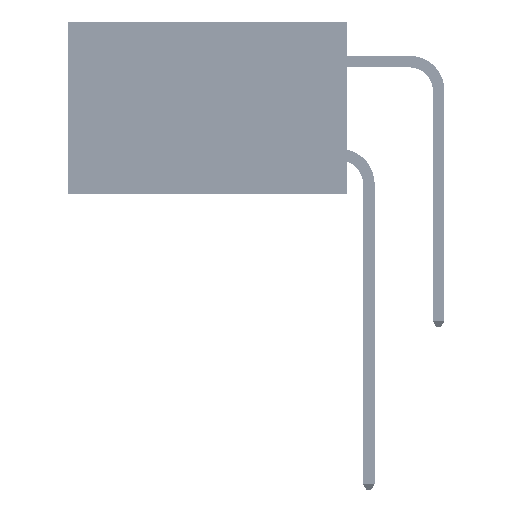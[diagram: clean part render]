
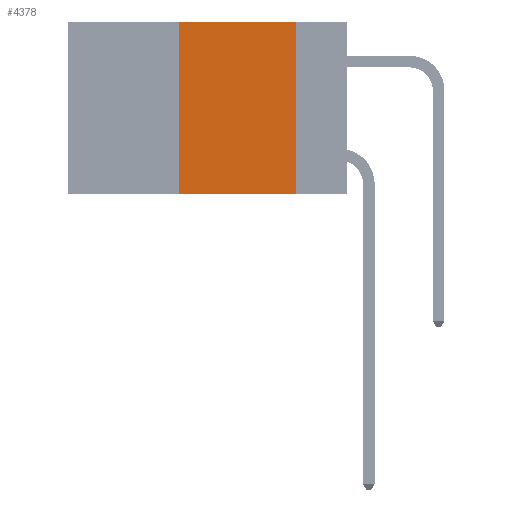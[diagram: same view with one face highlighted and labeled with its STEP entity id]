
A CAD part, left-side view. The second image highlights one B-rep face of the part: STEP entity #4378.
In plain terms, the highlighted planar face has unit normal (-1, 0, 0).
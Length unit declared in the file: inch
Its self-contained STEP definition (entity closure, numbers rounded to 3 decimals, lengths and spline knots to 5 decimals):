
#446 = AXIS2_PLACEMENT_3D ( 'NONE', #36371, #47798, #25046 ) ;
#1103 = CARTESIAN_POINT ( 'NONE',  ( 0., 0.11, 0. ) ) ;
#2057 = VERTEX_POINT ( 'NONE', #31451 ) ;
#3008 = ORIENTED_EDGE ( 'NONE', *, *, #12798, .T. ) ;
#3138 = EDGE_LOOP ( 'NONE', ( #3598, #27685, #30068, #3008 ) ) ;
#3598 = ORIENTED_EDGE ( 'NONE', *, *, #38986, .F. ) ;
#3683 = LINE ( 'NONE', #12601, #34325 ) ;
#4378 = ADVANCED_FACE ( 'NONE', ( #35462 ), #24865, .F. ) ;
#5439 = CARTESIAN_POINT ( 'NONE',  ( 0., 0.11, 0. ) ) ;
#5628 = EDGE_CURVE ( 'NONE', #45196, #2057, #17426, .T. ) ;
#8001 = CARTESIAN_POINT ( 'NONE',  ( 0., 0.11, -0.37 ) ) ;
#12601 = CARTESIAN_POINT ( 'NONE',  ( 0., 0.6, 0. ) ) ;
#12666 = DIRECTION ( 'NONE',  ( 0., 0., -1. ) ) ;
#12798 = EDGE_CURVE ( 'NONE', #45196, #36353, #18949, .T. ) ;
#17426 = LINE ( 'NONE', #43888, #26401 ) ;
#18949 = LINE ( 'NONE', #26692, #38016 ) ;
#20485 = CARTESIAN_POINT ( 'NONE',  ( 0., 0.36, -0.37 ) ) ;
#24865 = PLANE ( 'NONE',  #446 ) ;
#25046 = DIRECTION ( 'NONE',  ( 0., 0., -1. ) ) ;
#26401 = VECTOR ( 'NONE', #47703, 39.37008 ) ;
#26692 = CARTESIAN_POINT ( 'NONE',  ( 0., 0.6, -0.37 ) ) ;
#27685 = ORIENTED_EDGE ( 'NONE', *, *, #45122, .F. ) ;
#28437 = LINE ( 'NONE', #1103, #47453 ) ;
#30068 = ORIENTED_EDGE ( 'NONE', *, *, #5628, .F. ) ;
#30467 = VERTEX_POINT ( 'NONE', #5439 ) ;
#31451 = CARTESIAN_POINT ( 'NONE',  ( 0., 0.36, 0. ) ) ;
#34190 = DIRECTION ( 'NONE',  ( 0., -1., 0. ) ) ;
#34325 = VECTOR ( 'NONE', #39298, 39.37008 ) ;
#35462 = FACE_OUTER_BOUND ( 'NONE', #3138, .T. ) ;
#36353 = VERTEX_POINT ( 'NONE', #8001 ) ;
#36371 = CARTESIAN_POINT ( 'NONE',  ( 0., 0.6, 0. ) ) ;
#38016 = VECTOR ( 'NONE', #34190, 39.37008 ) ;
#38986 = EDGE_CURVE ( 'NONE', #30467, #36353, #28437, .T. ) ;
#39298 = DIRECTION ( 'NONE',  ( 0., -1., 0. ) ) ;
#43888 = CARTESIAN_POINT ( 'NONE',  ( 0., 0.36, 0. ) ) ;
#45122 = EDGE_CURVE ( 'NONE', #2057, #30467, #3683, .T. ) ;
#45196 = VERTEX_POINT ( 'NONE', #20485 ) ;
#47453 = VECTOR ( 'NONE', #12666, 39.37008 ) ;
#47703 = DIRECTION ( 'NONE',  ( 0., 0., 1. ) ) ;
#47798 = DIRECTION ( 'NONE',  ( 1., 0., 0. ) ) ;
